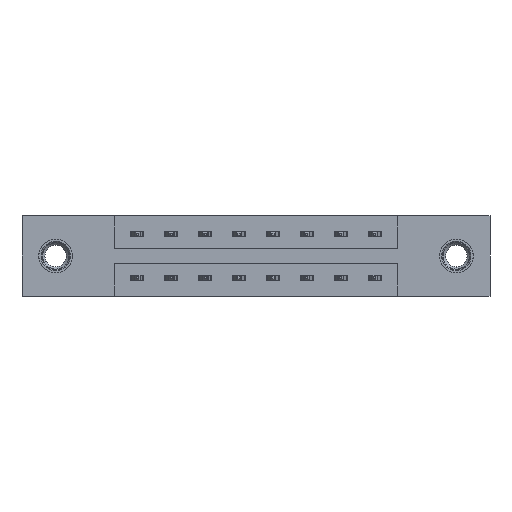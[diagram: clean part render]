
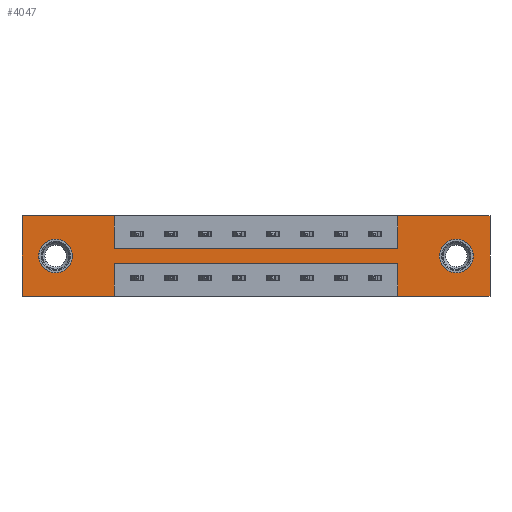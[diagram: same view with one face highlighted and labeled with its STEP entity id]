
A CAD part, front view. The second image highlights one B-rep face of the part: STEP entity #4047.
In plain terms, the highlighted planar face has unit normal (0, -1, 0).
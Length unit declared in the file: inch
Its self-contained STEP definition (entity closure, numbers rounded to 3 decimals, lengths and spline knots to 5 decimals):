
#153 = LINE ( 'NONE', #9675, #7371 ) ;
#161 = ORIENTED_EDGE ( 'NONE', *, *, #5927, .F. ) ;
#163 = VECTOR ( 'NONE', #1936, 39.37008 ) ;
#176 = LINE ( 'NONE', #4512, #7394 ) ;
#263 = LINE ( 'NONE', #3740, #4678 ) ;
#401 = CARTESIAN_POINT ( 'NONE',  ( 1.729, 0., 0. ) ) ;
#429 = FACE_OUTER_BOUND ( 'NONE', #10466, .T. ) ;
#443 = EDGE_CURVE ( 'NONE', #1139, #2194, #5810, .T. ) ;
#677 = ORIENTED_EDGE ( 'NONE', *, *, #4160, .F. ) ;
#714 = CARTESIAN_POINT ( 'NONE',  ( 1.729, 0., -0.22 ) ) ;
#847 = ORIENTED_EDGE ( 'NONE', *, *, #8020, .F. ) ;
#1139 = VERTEX_POINT ( 'NONE', #9159 ) ;
#1142 = EDGE_LOOP ( 'NONE', ( #9117, #10897 ) ) ;
#1365 = ORIENTED_EDGE ( 'NONE', *, *, #9440, .T. ) ;
#1652 = DIRECTION ( 'NONE',  ( 1., 0., 0. ) ) ;
#1807 = ORIENTED_EDGE ( 'NONE', *, *, #10173, .T. ) ;
#1827 = VERTEX_POINT ( 'NONE', #714 ) ;
#1936 = DIRECTION ( 'NONE',  ( 0., 0., -1. ) ) ;
#2057 = ORIENTED_EDGE ( 'NONE', *, *, #8348, .F. ) ;
#2160 = VERTEX_POINT ( 'NONE', #7511 ) ;
#2176 = CARTESIAN_POINT ( 'NONE',  ( 0.425, 0., -0.15 ) ) ;
#2194 = VERTEX_POINT ( 'NONE', #11046 ) ;
#2318 = DIRECTION ( 'NONE',  ( 0., 1., 0. ) ) ;
#2382 = LINE ( 'NONE', #4107, #163 ) ;
#2441 = CIRCLE ( 'NONE', #4288, 0.078 ) ;
#2513 = CARTESIAN_POINT ( 'NONE',  ( 2.154, 0., -0.37 ) ) ;
#2675 = VECTOR ( 'NONE', #8296, 39.37008 ) ;
#2740 = EDGE_CURVE ( 'NONE', #2816, #1139, #2382, .T. ) ;
#2796 = CARTESIAN_POINT ( 'NONE',  ( 0.425, 0., -0.22 ) ) ;
#2816 = VERTEX_POINT ( 'NONE', #5516 ) ;
#2914 = CIRCLE ( 'NONE', #5021, 0.078 ) ;
#2919 = DIRECTION ( 'NONE',  ( 0., 0., 1. ) ) ;
#3082 = CARTESIAN_POINT ( 'NONE',  ( 0.425, 0., -0.15 ) ) ;
#3337 = DIRECTION ( 'NONE',  ( 0., 0., -1. ) ) ;
#3392 = LINE ( 'NONE', #2796, #8065 ) ;
#3452 = DIRECTION ( 'NONE',  ( 0., 1., 0. ) ) ;
#3499 = CARTESIAN_POINT ( 'NONE',  ( 1.999, 0., -0.107 ) ) ;
#3581 = ORIENTED_EDGE ( 'NONE', *, *, #8050, .F. ) ;
#3740 = CARTESIAN_POINT ( 'NONE',  ( 1.729, 0., -0.37 ) ) ;
#3758 = VECTOR ( 'NONE', #2919, 39.37008 ) ;
#3931 = ORIENTED_EDGE ( 'NONE', *, *, #443, .F. ) ;
#3975 = PLANE ( 'NONE',  #5848 ) ;
#4046 = DIRECTION ( 'NONE',  ( 1., 0., 0. ) ) ;
#4047 = ADVANCED_FACE ( 'NONE', ( #9947, #7941, #429 ), #3975, .T. ) ;
#4107 = CARTESIAN_POINT ( 'NONE',  ( 0.425, 0., -0.37 ) ) ;
#4138 = VECTOR ( 'NONE', #4046, 39.37008 ) ;
#4160 = EDGE_CURVE ( 'NONE', #1827, #2816, #3392, .T. ) ;
#4288 = AXIS2_PLACEMENT_3D ( 'NONE', #8766, #8751, #8737 ) ;
#4304 = CARTESIAN_POINT ( 'NONE',  ( 0., 0., 0. ) ) ;
#4335 = VECTOR ( 'NONE', #7241, 39.37008 ) ;
#4437 = LINE ( 'NONE', #2176, #4138 ) ;
#4512 = CARTESIAN_POINT ( 'NONE',  ( 0., 0., 0. ) ) ;
#4538 = EDGE_CURVE ( 'NONE', #4545, #6538, #9263, .T. ) ;
#4545 = VERTEX_POINT ( 'NONE', #4304 ) ;
#4628 = LINE ( 'NONE', #5351, #9466 ) ;
#4678 = VECTOR ( 'NONE', #10978, 39.37008 ) ;
#4707 = CARTESIAN_POINT ( 'NONE',  ( 1.729, 0., -0.37 ) ) ;
#5021 = AXIS2_PLACEMENT_3D ( 'NONE', #5257, #11508, #6207 ) ;
#5079 = EDGE_LOOP ( 'NONE', ( #1807, #1365 ) ) ;
#5237 = VECTOR ( 'NONE', #7690, 39.37008 ) ;
#5257 = CARTESIAN_POINT ( 'NONE',  ( 1.999, 0., -0.185 ) ) ;
#5351 = CARTESIAN_POINT ( 'NONE',  ( 2.154, 0., 0. ) ) ;
#5460 = EDGE_CURVE ( 'NONE', #10666, #2160, #2441, .T. ) ;
#5470 = VERTEX_POINT ( 'NONE', #11415 ) ;
#5516 = CARTESIAN_POINT ( 'NONE',  ( 0.425, 0., -0.22 ) ) ;
#5545 = ORIENTED_EDGE ( 'NONE', *, *, #10412, .F. ) ;
#5810 = LINE ( 'NONE', #6099, #5237 ) ;
#5848 = AXIS2_PLACEMENT_3D ( 'NONE', #6730, #6195, #9740 ) ;
#5907 = EDGE_CURVE ( 'NONE', #8732, #7275, #4628, .T. ) ;
#5927 = EDGE_CURVE ( 'NONE', #7275, #6136, #6857, .T. ) ;
#6018 = CARTESIAN_POINT ( 'NONE',  ( 0.155, 0., -0.107 ) ) ;
#6099 = CARTESIAN_POINT ( 'NONE',  ( 0., 0., -0.37 ) ) ;
#6136 = VERTEX_POINT ( 'NONE', #4707 ) ;
#6195 = DIRECTION ( 'NONE',  ( 0., -1., 0. ) ) ;
#6207 = DIRECTION ( 'NONE',  ( 0., 0., -1. ) ) ;
#6296 = CARTESIAN_POINT ( 'NONE',  ( 0., 0., -0.37 ) ) ;
#6504 = ORIENTED_EDGE ( 'NONE', *, *, #2740, .F. ) ;
#6538 = VERTEX_POINT ( 'NONE', #7155 ) ;
#6730 = CARTESIAN_POINT ( 'NONE',  ( 0., 0., -0.37 ) ) ;
#6735 = ORIENTED_EDGE ( 'NONE', *, *, #8841, .F. ) ;
#6857 = LINE ( 'NONE', #6296, #4335 ) ;
#7155 = CARTESIAN_POINT ( 'NONE',  ( 0.425, 0., 0. ) ) ;
#7241 = DIRECTION ( 'NONE',  ( -1., 0., 0. ) ) ;
#7275 = VERTEX_POINT ( 'NONE', #2513 ) ;
#7371 = VECTOR ( 'NONE', #3337, 39.37008 ) ;
#7391 = CARTESIAN_POINT ( 'NONE',  ( 0., 0., 0. ) ) ;
#7394 = VECTOR ( 'NONE', #10843, 39.37008 ) ;
#7511 = CARTESIAN_POINT ( 'NONE',  ( 0.155, 0., -0.263 ) ) ;
#7569 = CARTESIAN_POINT ( 'NONE',  ( 1.729, 0., -0.15 ) ) ;
#7634 = AXIS2_PLACEMENT_3D ( 'NONE', #8954, #3452, #9826 ) ;
#7690 = DIRECTION ( 'NONE',  ( -1., 0., 0. ) ) ;
#7695 = VERTEX_POINT ( 'NONE', #3082 ) ;
#7760 = ORIENTED_EDGE ( 'NONE', *, *, #5907, .F. ) ;
#7941 = FACE_BOUND ( 'NONE', #1142, .T. ) ;
#7948 = CARTESIAN_POINT ( 'NONE',  ( 1.999, 0., -0.185 ) ) ;
#8020 = EDGE_CURVE ( 'NONE', #2194, #4545, #176, .T. ) ;
#8050 = EDGE_CURVE ( 'NONE', #11618, #8732, #9435, .T. ) ;
#8065 = VECTOR ( 'NONE', #11390, 39.37008 ) ;
#8296 = DIRECTION ( 'NONE',  ( 1., 0., 0. ) ) ;
#8348 = EDGE_CURVE ( 'NONE', #7695, #11129, #4437, .T. ) ;
#8399 = LINE ( 'NONE', #8481, #3758 ) ;
#8481 = CARTESIAN_POINT ( 'NONE',  ( 1.729, 0., 0. ) ) ;
#8732 = VERTEX_POINT ( 'NONE', #11275 ) ;
#8737 = DIRECTION ( 'NONE',  ( 0., 0., 1. ) ) ;
#8751 = DIRECTION ( 'NONE',  ( 0., 1., 0. ) ) ;
#8766 = CARTESIAN_POINT ( 'NONE',  ( 0.155, 0., -0.185 ) ) ;
#8777 = DIRECTION ( 'NONE',  ( 0., 0., -1. ) ) ;
#8841 = EDGE_CURVE ( 'NONE', #6538, #7695, #153, .T. ) ;
#8954 = CARTESIAN_POINT ( 'NONE',  ( 0.155, 0., -0.185 ) ) ;
#9117 = ORIENTED_EDGE ( 'NONE', *, *, #5460, .T. ) ;
#9159 = CARTESIAN_POINT ( 'NONE',  ( 0.425, 0., -0.37 ) ) ;
#9263 = LINE ( 'NONE', #10422, #11310 ) ;
#9435 = LINE ( 'NONE', #7391, #2675 ) ;
#9440 = EDGE_CURVE ( 'NONE', #5470, #10243, #10365, .T. ) ;
#9466 = VECTOR ( 'NONE', #11581, 39.37008 ) ;
#9516 = ORIENTED_EDGE ( 'NONE', *, *, #11138, .F. ) ;
#9675 = CARTESIAN_POINT ( 'NONE',  ( 0.425, 0., 0. ) ) ;
#9740 = DIRECTION ( 'NONE',  ( 0., 0., -1. ) ) ;
#9826 = DIRECTION ( 'NONE',  ( 0., 0., 1. ) ) ;
#9947 = FACE_BOUND ( 'NONE', #5079, .T. ) ;
#10173 = EDGE_CURVE ( 'NONE', #10243, #5470, #2914, .T. ) ;
#10243 = VERTEX_POINT ( 'NONE', #3499 ) ;
#10365 = CIRCLE ( 'NONE', #11121, 0.078 ) ;
#10412 = EDGE_CURVE ( 'NONE', #6136, #1827, #263, .T. ) ;
#10422 = CARTESIAN_POINT ( 'NONE',  ( 0., 0., 0. ) ) ;
#10466 = EDGE_LOOP ( 'NONE', ( #6504, #677, #5545, #161, #7760, #3581, #9516, #2057, #6735, #11006, #847, #3931 ) ) ;
#10666 = VERTEX_POINT ( 'NONE', #6018 ) ;
#10842 = CIRCLE ( 'NONE', #7634, 0.078 ) ;
#10843 = DIRECTION ( 'NONE',  ( 0., 0., 1. ) ) ;
#10897 = ORIENTED_EDGE ( 'NONE', *, *, #11770, .T. ) ;
#10978 = DIRECTION ( 'NONE',  ( 0., 0., 1. ) ) ;
#11006 = ORIENTED_EDGE ( 'NONE', *, *, #4538, .F. ) ;
#11046 = CARTESIAN_POINT ( 'NONE',  ( 0., 0., -0.37 ) ) ;
#11121 = AXIS2_PLACEMENT_3D ( 'NONE', #7948, #2318, #8777 ) ;
#11129 = VERTEX_POINT ( 'NONE', #7569 ) ;
#11138 = EDGE_CURVE ( 'NONE', #11129, #11618, #8399, .T. ) ;
#11275 = CARTESIAN_POINT ( 'NONE',  ( 2.154, 0., 0. ) ) ;
#11310 = VECTOR ( 'NONE', #1652, 39.37008 ) ;
#11390 = DIRECTION ( 'NONE',  ( -1., 0., 0. ) ) ;
#11415 = CARTESIAN_POINT ( 'NONE',  ( 1.999, 0., -0.263 ) ) ;
#11508 = DIRECTION ( 'NONE',  ( 0., 1., 0. ) ) ;
#11581 = DIRECTION ( 'NONE',  ( 0., 0., -1. ) ) ;
#11618 = VERTEX_POINT ( 'NONE', #401 ) ;
#11770 = EDGE_CURVE ( 'NONE', #2160, #10666, #10842, .T. ) ;
